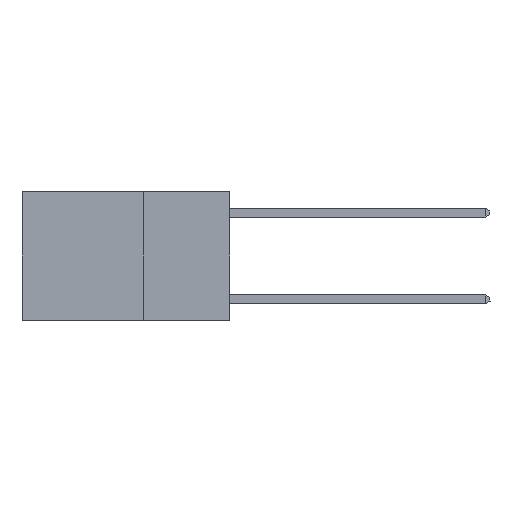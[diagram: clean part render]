
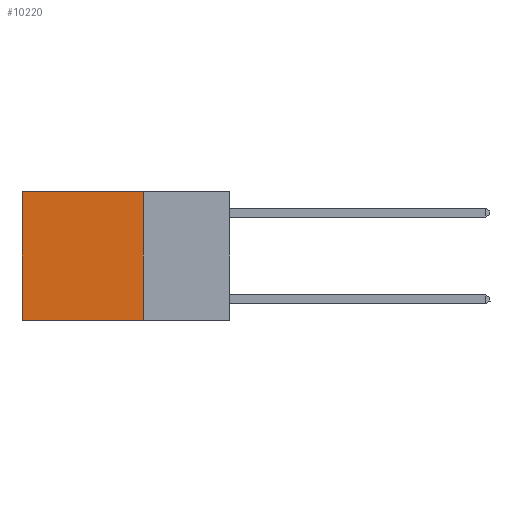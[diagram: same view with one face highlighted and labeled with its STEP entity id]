
A CAD part, left-side view. The second image highlights one B-rep face of the part: STEP entity #10220.
In plain terms, the highlighted planar face has unit normal (-1, 0, 0).
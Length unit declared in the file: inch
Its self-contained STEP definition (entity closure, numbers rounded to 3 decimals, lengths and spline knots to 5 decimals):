
#33 = LINE ( 'NONE', #717, #5072 ) ;
#176 = VECTOR ( 'NONE', #8151, 39.37008 ) ;
#608 = EDGE_CURVE ( 'NONE', #10456, #5478, #2268, .T. ) ;
#717 = CARTESIAN_POINT ( 'NONE',  ( 0.2625, 0.25, 0. ) ) ;
#1410 = ORIENTED_EDGE ( 'NONE', *, *, #5562, .T. ) ;
#1811 = EDGE_LOOP ( 'NONE', ( #5383, #9244, #12536, #1410 ) ) ;
#2268 = LINE ( 'NONE', #5882, #9607 ) ;
#2988 = EDGE_CURVE ( 'NONE', #6802, #5478, #3343, .T. ) ;
#3343 = LINE ( 'NONE', #3614, #5616 ) ;
#3614 = CARTESIAN_POINT ( 'NONE',  ( 0.2625, 0.6, 0. ) ) ;
#3829 = CARTESIAN_POINT ( 'NONE',  ( 0.2625, 0.25, 0. ) ) ;
#3856 = CARTESIAN_POINT ( 'NONE',  ( 0.2625, 0.25, 0. ) ) ;
#5072 = VECTOR ( 'NONE', #13120, 39.37008 ) ;
#5383 = ORIENTED_EDGE ( 'NONE', *, *, #2988, .T. ) ;
#5386 = DIRECTION ( 'NONE',  ( 1., 0., 0. ) ) ;
#5478 = VERTEX_POINT ( 'NONE', #8697 ) ;
#5562 = EDGE_CURVE ( 'NONE', #10868, #6802, #33, .T. ) ;
#5588 = DIRECTION ( 'NONE',  ( 0., 0., -1. ) ) ;
#5616 = VECTOR ( 'NONE', #5588, 39.37008 ) ;
#5882 = CARTESIAN_POINT ( 'NONE',  ( 0.2625, 0.25, -0.37 ) ) ;
#6255 = DIRECTION ( 'NONE',  ( 0., 0., -1. ) ) ;
#6802 = VERTEX_POINT ( 'NONE', #10172 ) ;
#6944 = DIRECTION ( 'NONE',  ( 0., 1., 0. ) ) ;
#7318 = PLANE ( 'NONE',  #11128 ) ;
#8151 = DIRECTION ( 'NONE',  ( 0., 0., -1. ) ) ;
#8457 = FACE_OUTER_BOUND ( 'NONE', #1811, .T. ) ;
#8697 = CARTESIAN_POINT ( 'NONE',  ( 0.2625, 0.6, -0.37 ) ) ;
#9244 = ORIENTED_EDGE ( 'NONE', *, *, #608, .F. ) ;
#9423 = CARTESIAN_POINT ( 'NONE',  ( 0.2625, 0.25, 0. ) ) ;
#9607 = VECTOR ( 'NONE', #6944, 39.37008 ) ;
#9975 = EDGE_CURVE ( 'NONE', #10868, #10456, #11564, .T. ) ;
#10172 = CARTESIAN_POINT ( 'NONE',  ( 0.2625, 0.6, 0. ) ) ;
#10220 = ADVANCED_FACE ( 'NONE', ( #8457 ), #7318, .F. ) ;
#10456 = VERTEX_POINT ( 'NONE', #12011 ) ;
#10868 = VERTEX_POINT ( 'NONE', #3829 ) ;
#11128 = AXIS2_PLACEMENT_3D ( 'NONE', #9423, #5386, #6255 ) ;
#11564 = LINE ( 'NONE', #3856, #176 ) ;
#12011 = CARTESIAN_POINT ( 'NONE',  ( 0.2625, 0.25, -0.37 ) ) ;
#12536 = ORIENTED_EDGE ( 'NONE', *, *, #9975, .F. ) ;
#13120 = DIRECTION ( 'NONE',  ( 0., 1., 0. ) ) ;
